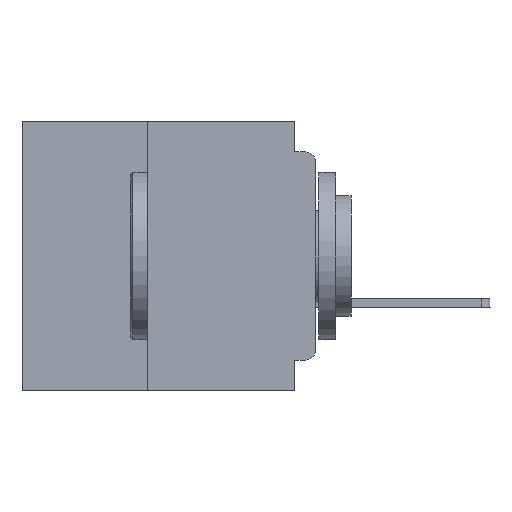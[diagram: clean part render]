
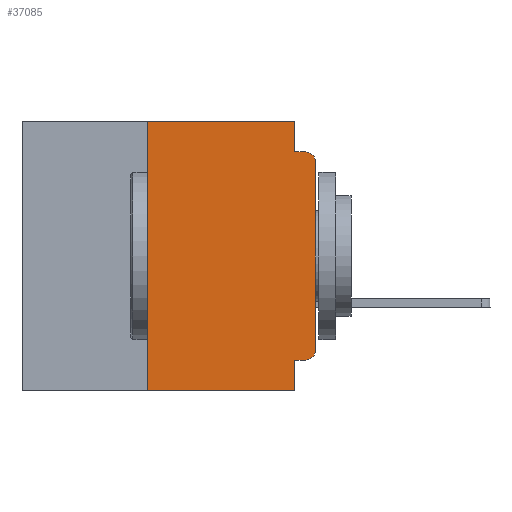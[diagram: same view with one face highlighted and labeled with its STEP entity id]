
A CAD part, left-side view. The second image highlights one B-rep face of the part: STEP entity #37085.
In plain terms, the highlighted planar face has unit normal (-1, 0, 0).
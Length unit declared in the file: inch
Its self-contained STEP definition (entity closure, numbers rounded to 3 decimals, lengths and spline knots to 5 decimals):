
#1095 = CARTESIAN_POINT ( 'NONE',  ( 0., 0.437, -0.4 ) ) ;
#5991 = LINE ( 'NONE', #53122, #31537 ) ;
#6983 = EDGE_CURVE ( 'NONE', #36737, #52102, #38981, .T. ) ;
#9175 = EDGE_CURVE ( 'NONE', #18076, #34551, #34720, .T. ) ;
#11512 = VECTOR ( 'NONE', #25093, 39.37008 ) ;
#11636 = CARTESIAN_POINT ( 'NONE',  ( 0., 0.031, 0. ) ) ;
#11729 = EDGE_CURVE ( 'NONE', #12579, #40746, #13584, .T. ) ;
#11820 = VECTOR ( 'NONE', #29282, 39.37008 ) ;
#12579 = VERTEX_POINT ( 'NONE', #13921 ) ;
#13426 = LINE ( 'NONE', #24119, #11820 ) ;
#13584 = LINE ( 'NONE', #58035, #37558 ) ;
#13921 = CARTESIAN_POINT ( 'NONE',  ( 0., 0., -0.34 ) ) ;
#15220 = DIRECTION ( 'NONE',  ( -1., 0., 0. ) ) ;
#15335 = CARTESIAN_POINT ( 'NONE',  ( 0., 0., -0.045 ) ) ;
#15636 = CARTESIAN_POINT ( 'NONE',  ( 0., 0.031, -0.355 ) ) ;
#16366 = CARTESIAN_POINT ( 'NONE',  ( 0., 0.015, -0.06 ) ) ;
#16543 = CARTESIAN_POINT ( 'NONE',  ( 0., 0.031, 0. ) ) ;
#16771 = DIRECTION ( 'NONE',  ( 0., 0., -1. ) ) ;
#17083 = CIRCLE ( 'NONE', #43326, 0.015 ) ;
#17183 = LINE ( 'NONE', #11636, #30784 ) ;
#18076 = VERTEX_POINT ( 'NONE', #60917 ) ;
#18211 = LINE ( 'NONE', #1095, #45399 ) ;
#18579 = DIRECTION ( 'NONE',  ( 0., 1., 0. ) ) ;
#19484 = CARTESIAN_POINT ( 'NONE',  ( 0., 0.031, -0.4 ) ) ;
#19711 = ORIENTED_EDGE ( 'NONE', *, *, #45296, .F. ) ;
#20703 = EDGE_CURVE ( 'NONE', #24851, #36737, #17183, .T. ) ;
#21296 = CARTESIAN_POINT ( 'NONE',  ( 0., 0., -0.06 ) ) ;
#21513 = DIRECTION ( 'NONE',  ( 0., 0., -1. ) ) ;
#22157 = VERTEX_POINT ( 'NONE', #54127 ) ;
#22534 = CARTESIAN_POINT ( 'NONE',  ( 0., 0.015, -0.045 ) ) ;
#24119 = CARTESIAN_POINT ( 'NONE',  ( 0., 0.031, -0.4 ) ) ;
#24851 = VERTEX_POINT ( 'NONE', #16543 ) ;
#24959 = CIRCLE ( 'NONE', #37635, 0.015 ) ;
#25093 = DIRECTION ( 'NONE',  ( 0., 0., 1. ) ) ;
#26659 = LINE ( 'NONE', #40322, #11512 ) ;
#26911 = VECTOR ( 'NONE', #50871, 39.37008 ) ;
#26954 = ORIENTED_EDGE ( 'NONE', *, *, #40754, .T. ) ;
#27373 = DIRECTION ( 'NONE',  ( 0., 0., 1. ) ) ;
#27411 = DIRECTION ( 'NONE',  ( 0., -1., 0. ) ) ;
#28657 = CARTESIAN_POINT ( 'NONE',  ( 0., 0.25, 0. ) ) ;
#29282 = DIRECTION ( 'NONE',  ( 0., 0., -1. ) ) ;
#30177 = VERTEX_POINT ( 'NONE', #19484 ) ;
#30503 = ORIENTED_EDGE ( 'NONE', *, *, #66175, .T. ) ;
#30784 = VECTOR ( 'NONE', #16771, 39.37008 ) ;
#31537 = VECTOR ( 'NONE', #27411, 39.37008 ) ;
#31666 = DIRECTION ( 'NONE',  ( 0., -1., 0. ) ) ;
#32800 = DIRECTION ( 'NONE',  ( 0., 0., -1. ) ) ;
#34551 = VERTEX_POINT ( 'NONE', #15636 ) ;
#34720 = LINE ( 'NONE', #59452, #60307 ) ;
#36737 = VERTEX_POINT ( 'NONE', #54692 ) ;
#37065 = ORIENTED_EDGE ( 'NONE', *, *, #6983, .F. ) ;
#37085 = ADVANCED_FACE ( 'NONE', ( #62245 ), #58297, .F. ) ;
#37558 = VECTOR ( 'NONE', #27373, 39.37008 ) ;
#37635 = AXIS2_PLACEMENT_3D ( 'NONE', #45832, #15220, #50974 ) ;
#38539 = ORIENTED_EDGE ( 'NONE', *, *, #11729, .T. ) ;
#38981 = LINE ( 'NONE', #15335, #26911 ) ;
#40322 = CARTESIAN_POINT ( 'NONE',  ( 0., 0.25, -0.4 ) ) ;
#40578 = EDGE_CURVE ( 'NONE', #22157, #63116, #26659, .T. ) ;
#40746 = VERTEX_POINT ( 'NONE', #21296 ) ;
#40754 = EDGE_CURVE ( 'NONE', #40746, #52102, #17083, .T. ) ;
#41518 = EDGE_CURVE ( 'NONE', #63116, #24851, #5991, .T. ) ;
#43326 = AXIS2_PLACEMENT_3D ( 'NONE', #16366, #52115, #21513 ) ;
#43372 = EDGE_LOOP ( 'NONE', ( #38539, #26954, #37065, #62042, #64016, #49898, #44951, #19711, #46943, #30503 ) ) ;
#44951 = ORIENTED_EDGE ( 'NONE', *, *, #47244, .T. ) ;
#45296 = EDGE_CURVE ( 'NONE', #34551, #30177, #13426, .T. ) ;
#45399 = VECTOR ( 'NONE', #31666, 39.37008 ) ;
#45832 = CARTESIAN_POINT ( 'NONE',  ( 0., 0.015, -0.34 ) ) ;
#46173 = AXIS2_PLACEMENT_3D ( 'NONE', #53121, #63383, #32800 ) ;
#46943 = ORIENTED_EDGE ( 'NONE', *, *, #9175, .F. ) ;
#47244 = EDGE_CURVE ( 'NONE', #22157, #30177, #18211, .T. ) ;
#49898 = ORIENTED_EDGE ( 'NONE', *, *, #40578, .F. ) ;
#50871 = DIRECTION ( 'NONE',  ( 0., -1., 0. ) ) ;
#50974 = DIRECTION ( 'NONE',  ( 0., 0., -1. ) ) ;
#52102 = VERTEX_POINT ( 'NONE', #22534 ) ;
#52115 = DIRECTION ( 'NONE',  ( -1., 0., 0. ) ) ;
#53121 = CARTESIAN_POINT ( 'NONE',  ( 0., 0.437, 0. ) ) ;
#53122 = CARTESIAN_POINT ( 'NONE',  ( 0., 0.437, 0. ) ) ;
#54127 = CARTESIAN_POINT ( 'NONE',  ( 0., 0.25, -0.4 ) ) ;
#54692 = CARTESIAN_POINT ( 'NONE',  ( 0., 0.031, -0.045 ) ) ;
#58035 = CARTESIAN_POINT ( 'NONE',  ( 0., 0., 0. ) ) ;
#58297 = PLANE ( 'NONE',  #46173 ) ;
#59452 = CARTESIAN_POINT ( 'NONE',  ( 0., 0., -0.355 ) ) ;
#60307 = VECTOR ( 'NONE', #18579, 39.37008 ) ;
#60917 = CARTESIAN_POINT ( 'NONE',  ( 0., 0.015, -0.355 ) ) ;
#62042 = ORIENTED_EDGE ( 'NONE', *, *, #20703, .F. ) ;
#62245 = FACE_OUTER_BOUND ( 'NONE', #43372, .T. ) ;
#63116 = VERTEX_POINT ( 'NONE', #28657 ) ;
#63383 = DIRECTION ( 'NONE',  ( 1., 0., 0. ) ) ;
#64016 = ORIENTED_EDGE ( 'NONE', *, *, #41518, .F. ) ;
#66175 = EDGE_CURVE ( 'NONE', #18076, #12579, #24959, .T. ) ;
